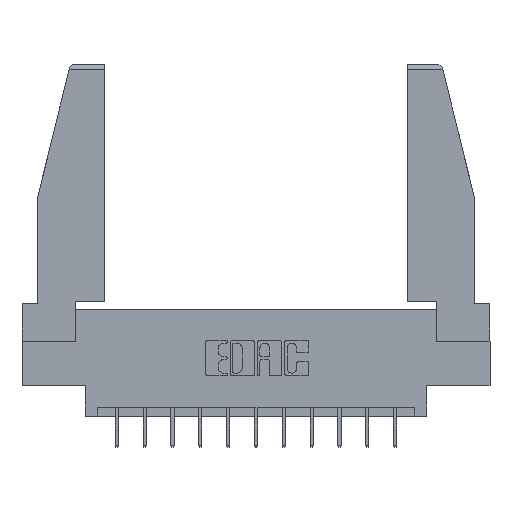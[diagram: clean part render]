
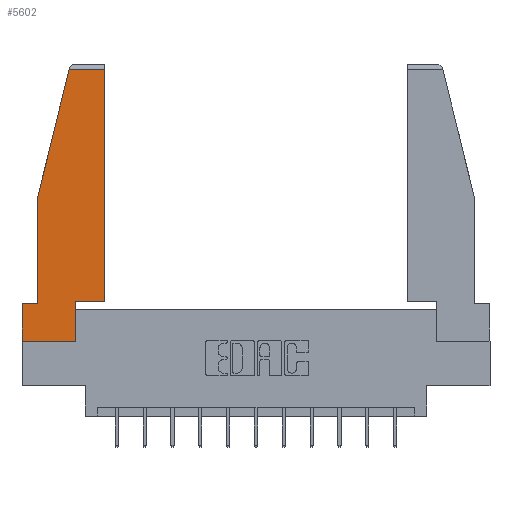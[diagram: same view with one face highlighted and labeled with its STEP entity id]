
A CAD part, top view. The second image highlights one B-rep face of the part: STEP entity #5602.
In plain terms, the highlighted planar face has unit normal (0, 0, 1).
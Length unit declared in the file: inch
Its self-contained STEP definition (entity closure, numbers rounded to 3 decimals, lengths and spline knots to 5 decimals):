
#117 = VERTEX_POINT ( 'NONE', #10742 ) ;
#545 = VERTEX_POINT ( 'NONE', #4952 ) ;
#551 = VECTOR ( 'NONE', #14609, 39.37008 ) ;
#623 = DIRECTION ( 'NONE',  ( -0.239, -0.971, 0. ) ) ;
#659 = CARTESIAN_POINT ( 'NONE',  ( 0.2636, 1.52, 0. ) ) ;
#696 = EDGE_CURVE ( 'NONE', #13409, #545, #12271, .T. ) ;
#793 = CARTESIAN_POINT ( 'NONE',  ( 0.086, 0.8, 0. ) ) ;
#807 = CARTESIAN_POINT ( 'NONE',  ( 0., 0., 0. ) ) ;
#1360 = VECTOR ( 'NONE', #12449, 39.37008 ) ;
#1563 = CARTESIAN_POINT ( 'NONE',  ( 0., 0.21, 0. ) ) ;
#1806 = ORIENTED_EDGE ( 'NONE', *, *, #14816, .T. ) ;
#2096 = LINE ( 'NONE', #14582, #6873 ) ;
#2146 = VECTOR ( 'NONE', #3083, 39.37008 ) ;
#2587 = FACE_OUTER_BOUND ( 'NONE', #7060, .T. ) ;
#2877 = LINE ( 'NONE', #793, #2146 ) ;
#3076 = VECTOR ( 'NONE', #623, 39.37008 ) ;
#3083 = DIRECTION ( 'NONE',  ( 0., -1., 0. ) ) ;
#4163 = CARTESIAN_POINT ( 'NONE',  ( 0.297, 0., 0. ) ) ;
#4195 = AXIS2_PLACEMENT_3D ( 'NONE', #11907, #10901, #10845 ) ;
#4546 = VERTEX_POINT ( 'NONE', #13104 ) ;
#4952 = CARTESIAN_POINT ( 'NONE',  ( 0.297, 0.223, 0. ) ) ;
#4964 = VERTEX_POINT ( 'NONE', #4988 ) ;
#4988 = CARTESIAN_POINT ( 'NONE',  ( 0.461, 0.223, 0. ) ) ;
#5602 = ADVANCED_FACE ( 'NONE', ( #2587 ), #13017, .T. ) ;
#5986 = ORIENTED_EDGE ( 'NONE', *, *, #9309, .T. ) ;
#6164 = EDGE_CURVE ( 'NONE', #4546, #11019, #2877, .T. ) ;
#6284 = LINE ( 'NONE', #1563, #551 ) ;
#6417 = ORIENTED_EDGE ( 'NONE', *, *, #12018, .T. ) ;
#6438 = DIRECTION ( 'NONE',  ( 0., 1., 0. ) ) ;
#6643 = VERTEX_POINT ( 'NONE', #10965 ) ;
#6873 = VECTOR ( 'NONE', #7607, 39.37008 ) ;
#7020 = LINE ( 'NONE', #807, #14107 ) ;
#7060 = EDGE_LOOP ( 'NONE', ( #13300, #7112, #5986, #8447, #6417, #15211, #13966, #8214, #1806 ) ) ;
#7112 = ORIENTED_EDGE ( 'NONE', *, *, #10082, .T. ) ;
#7190 = DIRECTION ( 'NONE',  ( 0., -1., 0. ) ) ;
#7607 = DIRECTION ( 'NONE',  ( -1., 0., 0. ) ) ;
#7662 = CARTESIAN_POINT ( 'NONE',  ( 0.271, 1.55, 0. ) ) ;
#7707 = LINE ( 'NONE', #10757, #13738 ) ;
#7855 = CARTESIAN_POINT ( 'NONE',  ( 0.086, 0.21, 0. ) ) ;
#8214 = ORIENTED_EDGE ( 'NONE', *, *, #696, .T. ) ;
#8447 = ORIENTED_EDGE ( 'NONE', *, *, #6164, .T. ) ;
#8464 = EDGE_CURVE ( 'NONE', #9597, #6643, #7707, .T. ) ;
#9038 = VECTOR ( 'NONE', #12644, 39.37008 ) ;
#9309 = EDGE_CURVE ( 'NONE', #13370, #4546, #13147, .T. ) ;
#9389 = LINE ( 'NONE', #13320, #9038 ) ;
#9597 = VERTEX_POINT ( 'NONE', #15134 ) ;
#10082 = EDGE_CURVE ( 'NONE', #117, #13370, #2096, .T. ) ;
#10309 = DIRECTION ( 'NONE',  ( 1., 0., 0. ) ) ;
#10742 = CARTESIAN_POINT ( 'NONE',  ( 0.461, 1.52, 0. ) ) ;
#10757 = CARTESIAN_POINT ( 'NONE',  ( 0., 0.21, 0. ) ) ;
#10845 = DIRECTION ( 'NONE',  ( 1., 0., 0. ) ) ;
#10901 = DIRECTION ( 'NONE',  ( 0., 0., 1. ) ) ;
#10965 = CARTESIAN_POINT ( 'NONE',  ( 0., 0., 0. ) ) ;
#11019 = VERTEX_POINT ( 'NONE', #7855 ) ;
#11631 = CARTESIAN_POINT ( 'NONE',  ( 0.297, 0., 0. ) ) ;
#11907 = CARTESIAN_POINT ( 'NONE',  ( 0., 0., 0. ) ) ;
#12018 = EDGE_CURVE ( 'NONE', #11019, #9597, #6284, .T. ) ;
#12032 = EDGE_CURVE ( 'NONE', #4964, #117, #9389, .T. ) ;
#12129 = EDGE_CURVE ( 'NONE', #6643, #13409, #7020, .T. ) ;
#12271 = LINE ( 'NONE', #4163, #14083 ) ;
#12449 = DIRECTION ( 'NONE',  ( 1., 0., 0. ) ) ;
#12534 = LINE ( 'NONE', #14719, #1360 ) ;
#12644 = DIRECTION ( 'NONE',  ( 0., 1., 0. ) ) ;
#13017 = PLANE ( 'NONE',  #4195 ) ;
#13104 = CARTESIAN_POINT ( 'NONE',  ( 0.086, 0.8, 0. ) ) ;
#13147 = LINE ( 'NONE', #7662, #3076 ) ;
#13300 = ORIENTED_EDGE ( 'NONE', *, *, #12032, .T. ) ;
#13320 = CARTESIAN_POINT ( 'NONE',  ( 0.461, 0.223, 0. ) ) ;
#13370 = VERTEX_POINT ( 'NONE', #659 ) ;
#13409 = VERTEX_POINT ( 'NONE', #11631 ) ;
#13738 = VECTOR ( 'NONE', #7190, 39.37008 ) ;
#13966 = ORIENTED_EDGE ( 'NONE', *, *, #12129, .T. ) ;
#14083 = VECTOR ( 'NONE', #6438, 39.37008 ) ;
#14107 = VECTOR ( 'NONE', #10309, 39.37008 ) ;
#14582 = CARTESIAN_POINT ( 'NONE',  ( 0., 1.52, 0. ) ) ;
#14609 = DIRECTION ( 'NONE',  ( -1., 0., 0. ) ) ;
#14719 = CARTESIAN_POINT ( 'NONE',  ( 0.297, 0.223, 0. ) ) ;
#14816 = EDGE_CURVE ( 'NONE', #545, #4964, #12534, .T. ) ;
#15134 = CARTESIAN_POINT ( 'NONE',  ( 0., 0.21, 0. ) ) ;
#15211 = ORIENTED_EDGE ( 'NONE', *, *, #8464, .T. ) ;
